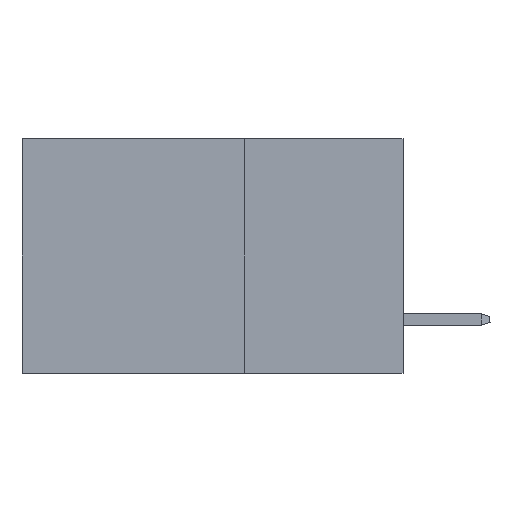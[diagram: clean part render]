
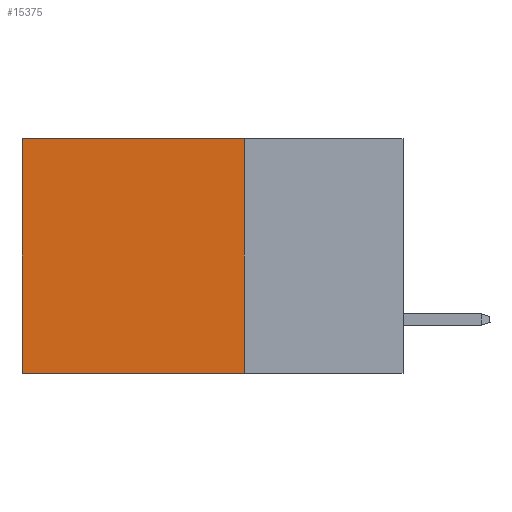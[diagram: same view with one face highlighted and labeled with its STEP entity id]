
A CAD part, left-side view. The second image highlights one B-rep face of the part: STEP entity #15375.
In plain terms, the highlighted planar face has unit normal (-1, 0, 0).
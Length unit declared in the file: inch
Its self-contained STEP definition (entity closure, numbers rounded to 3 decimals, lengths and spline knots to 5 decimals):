
#140 = VECTOR ( 'NONE', #8820, 39.37008 ) ;
#1136 = ORIENTED_EDGE ( 'NONE', *, *, #9589, .F. ) ;
#1189 = CARTESIAN_POINT ( 'NONE',  ( 0.2875, 0.6, 0. ) ) ;
#1727 = VECTOR ( 'NONE', #16411, 39.37008 ) ;
#2461 = LINE ( 'NONE', #1189, #1727 ) ;
#2544 = CARTESIAN_POINT ( 'NONE',  ( 0.2875, 0.25, 0. ) ) ;
#2851 = DIRECTION ( 'NONE',  ( 1., 0., 0. ) ) ;
#2970 = ORIENTED_EDGE ( 'NONE', *, *, #8883, .T. ) ;
#3486 = CARTESIAN_POINT ( 'NONE',  ( 0.2875, 0.25, 0. ) ) ;
#5603 = CARTESIAN_POINT ( 'NONE',  ( 0.2875, 0.6, -0.37 ) ) ;
#6583 = ORIENTED_EDGE ( 'NONE', *, *, #6629, .T. ) ;
#6629 = EDGE_CURVE ( 'NONE', #7361, #15744, #15120, .T. ) ;
#7053 = PLANE ( 'NONE',  #8659 ) ;
#7210 = CARTESIAN_POINT ( 'NONE',  ( 0.2875, 0.25, 0. ) ) ;
#7361 = VERTEX_POINT ( 'NONE', #3486 ) ;
#7913 = VERTEX_POINT ( 'NONE', #14253 ) ;
#8594 = VERTEX_POINT ( 'NONE', #5603 ) ;
#8659 = AXIS2_PLACEMENT_3D ( 'NONE', #10002, #2851, #11039 ) ;
#8820 = DIRECTION ( 'NONE',  ( 0., 1., 0. ) ) ;
#8883 = EDGE_CURVE ( 'NONE', #15744, #8594, #2461, .T. ) ;
#8960 = ORIENTED_EDGE ( 'NONE', *, *, #14265, .F. ) ;
#8961 = EDGE_LOOP ( 'NONE', ( #2970, #8960, #1136, #6583 ) ) ;
#9589 = EDGE_CURVE ( 'NONE', #7361, #7913, #14463, .T. ) ;
#10002 = CARTESIAN_POINT ( 'NONE',  ( 0.2875, 0.25, 0. ) ) ;
#11039 = DIRECTION ( 'NONE',  ( 0., 0., -1. ) ) ;
#11307 = FACE_OUTER_BOUND ( 'NONE', #8961, .T. ) ;
#11492 = VECTOR ( 'NONE', #13762, 39.37008 ) ;
#11630 = DIRECTION ( 'NONE',  ( 0., 0., -1. ) ) ;
#13212 = VECTOR ( 'NONE', #11630, 39.37008 ) ;
#13762 = DIRECTION ( 'NONE',  ( 0., 1., 0. ) ) ;
#14253 = CARTESIAN_POINT ( 'NONE',  ( 0.2875, 0.25, -0.37 ) ) ;
#14264 = CARTESIAN_POINT ( 'NONE',  ( 0.2875, 0.6, 0. ) ) ;
#14265 = EDGE_CURVE ( 'NONE', #7913, #8594, #14405, .T. ) ;
#14405 = LINE ( 'NONE', #14512, #140 ) ;
#14463 = LINE ( 'NONE', #7210, #13212 ) ;
#14512 = CARTESIAN_POINT ( 'NONE',  ( 0.2875, 0.25, -0.37 ) ) ;
#15120 = LINE ( 'NONE', #2544, #11492 ) ;
#15375 = ADVANCED_FACE ( 'NONE', ( #11307 ), #7053, .F. ) ;
#15744 = VERTEX_POINT ( 'NONE', #14264 ) ;
#16411 = DIRECTION ( 'NONE',  ( 0., 0., -1. ) ) ;
